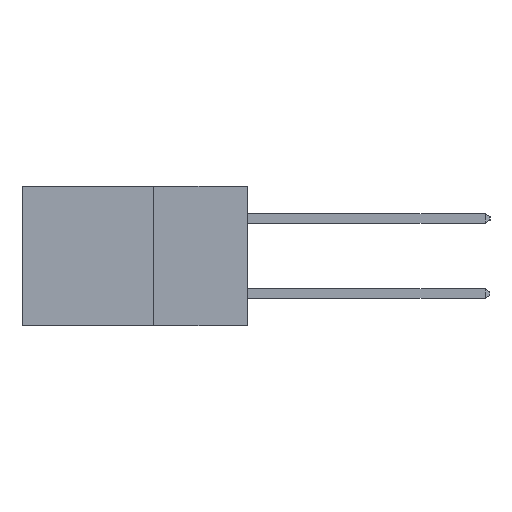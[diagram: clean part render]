
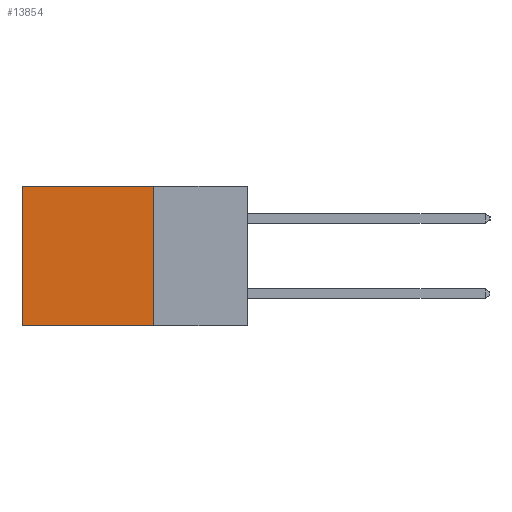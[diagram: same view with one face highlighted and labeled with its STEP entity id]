
A CAD part, left-side view. The second image highlights one B-rep face of the part: STEP entity #13854.
In plain terms, the highlighted planar face has unit normal (-1, 0, 0).
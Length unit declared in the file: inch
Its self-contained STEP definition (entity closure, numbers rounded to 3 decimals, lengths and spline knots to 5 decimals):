
#926 = CARTESIAN_POINT ( 'NONE',  ( 0.2615, 0.6, 0. ) ) ;
#1126 = CARTESIAN_POINT ( 'NONE',  ( 0.2615, 0.25, -0.37 ) ) ;
#1227 = LINE ( 'NONE', #16636, #18404 ) ;
#1645 = VERTEX_POINT ( 'NONE', #926 ) ;
#2133 = DIRECTION ( 'NONE',  ( 0., 1., 0. ) ) ;
#3394 = LINE ( 'NONE', #12780, #13812 ) ;
#4887 = DIRECTION ( 'NONE',  ( 0., 0., -1. ) ) ;
#5731 = AXIS2_PLACEMENT_3D ( 'NONE', #6260, #20593, #8333 ) ;
#6260 = CARTESIAN_POINT ( 'NONE',  ( 0.2615, 0.25, -0.37 ) ) ;
#7451 = VERTEX_POINT ( 'NONE', #14224 ) ;
#7477 = DIRECTION ( 'NONE',  ( 0., 1., 0. ) ) ;
#8030 = EDGE_CURVE ( 'NONE', #1645, #7451, #3394, .T. ) ;
#8333 = DIRECTION ( 'NONE',  ( 0., 0., -1. ) ) ;
#8358 = VECTOR ( 'NONE', #7477, 39.37008 ) ;
#10827 = EDGE_CURVE ( 'NONE', #11254, #7451, #26453, .T. ) ;
#11254 = VERTEX_POINT ( 'NONE', #14865 ) ;
#11623 = ORIENTED_EDGE ( 'NONE', *, *, #10827, .F. ) ;
#11722 = ORIENTED_EDGE ( 'NONE', *, *, #20665, .F. ) ;
#12415 = EDGE_LOOP ( 'NONE', ( #24258, #11623, #11722, #15570 ) ) ;
#12780 = CARTESIAN_POINT ( 'NONE',  ( 0.2615, 0.6, -0.37 ) ) ;
#13102 = LINE ( 'NONE', #15208, #13728 ) ;
#13728 = VECTOR ( 'NONE', #4887, 39.37008 ) ;
#13812 = VECTOR ( 'NONE', #14820, 39.37008 ) ;
#13854 = ADVANCED_FACE ( 'NONE', ( #20973 ), #26515, .F. ) ;
#14224 = CARTESIAN_POINT ( 'NONE',  ( 0.2615, 0.6, -0.37 ) ) ;
#14820 = DIRECTION ( 'NONE',  ( 0., 0., -1. ) ) ;
#14865 = CARTESIAN_POINT ( 'NONE',  ( 0.2615, 0.25, -0.37 ) ) ;
#15208 = CARTESIAN_POINT ( 'NONE',  ( 0.2615, 0.25, -0.37 ) ) ;
#15570 = ORIENTED_EDGE ( 'NONE', *, *, #25688, .T. ) ;
#16636 = CARTESIAN_POINT ( 'NONE',  ( 0.2615, 0.25, 0. ) ) ;
#18404 = VECTOR ( 'NONE', #2133, 39.37008 ) ;
#19417 = CARTESIAN_POINT ( 'NONE',  ( 0.2615, 0.25, 0. ) ) ;
#20593 = DIRECTION ( 'NONE',  ( 1., 0., 0. ) ) ;
#20665 = EDGE_CURVE ( 'NONE', #21996, #11254, #13102, .T. ) ;
#20973 = FACE_OUTER_BOUND ( 'NONE', #12415, .T. ) ;
#21996 = VERTEX_POINT ( 'NONE', #19417 ) ;
#24258 = ORIENTED_EDGE ( 'NONE', *, *, #8030, .T. ) ;
#25688 = EDGE_CURVE ( 'NONE', #21996, #1645, #1227, .T. ) ;
#26453 = LINE ( 'NONE', #1126, #8358 ) ;
#26515 = PLANE ( 'NONE',  #5731 ) ;
